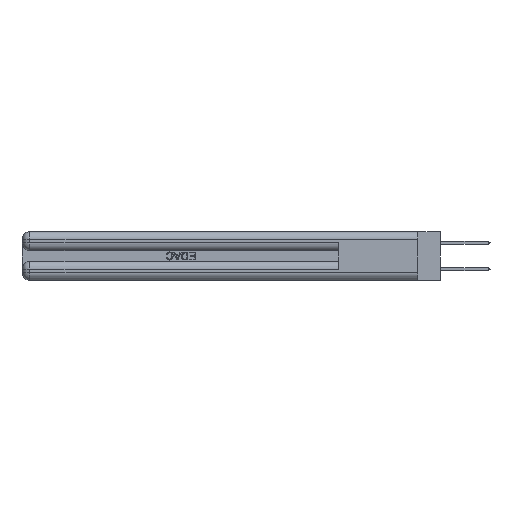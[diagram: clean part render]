
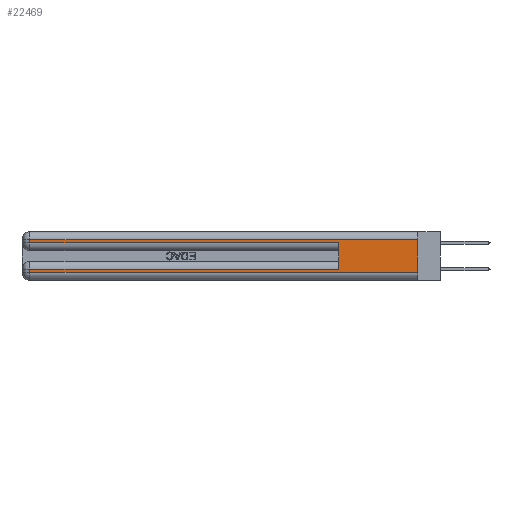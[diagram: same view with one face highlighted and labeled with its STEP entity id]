
A CAD part, left-side view. The second image highlights one B-rep face of the part: STEP entity #22469.
In plain terms, the highlighted planar face has unit normal (-1, 0, 0).
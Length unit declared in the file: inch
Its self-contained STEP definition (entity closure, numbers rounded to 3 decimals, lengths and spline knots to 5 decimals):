
#849 = DIRECTION ( 'NONE',  ( 0., 0., -1. ) ) ;
#931 = VECTOR ( 'NONE', #8853, 39.37008 ) ;
#965 = VERTEX_POINT ( 'NONE', #5379 ) ;
#1488 = CARTESIAN_POINT ( 'NONE',  ( 0., 0.6, 0.285 ) ) ;
#1806 = DIRECTION ( 'NONE',  ( 0., 1., 0. ) ) ;
#2777 = ORIENTED_EDGE ( 'NONE', *, *, #23682, .F. ) ;
#2875 = VERTEX_POINT ( 'NONE', #8921 ) ;
#2984 = DIRECTION ( 'NONE',  ( 0., 0., -1. ) ) ;
#4724 = VECTOR ( 'NONE', #29897, 39.37008 ) ;
#5170 = EDGE_CURVE ( 'NONE', #48050, #49299, #44335, .T. ) ;
#5379 = CARTESIAN_POINT ( 'NONE',  ( 0., 2.94, 0.285 ) ) ;
#5836 = CARTESIAN_POINT ( 'NONE',  ( 0., 0., 0.37 ) ) ;
#6632 = CARTESIAN_POINT ( 'NONE',  ( 0., 2.94, 0.37 ) ) ;
#6850 = VERTEX_POINT ( 'NONE', #25359 ) ;
#8327 = LINE ( 'NONE', #14644, #4724 ) ;
#8853 = DIRECTION ( 'NONE',  ( 0., 0., 1. ) ) ;
#8921 = CARTESIAN_POINT ( 'NONE',  ( 0., 2.94, 0.085 ) ) ;
#9682 = PLANE ( 'NONE',  #49146 ) ;
#9744 = LINE ( 'NONE', #6632, #49109 ) ;
#12824 = EDGE_CURVE ( 'NONE', #6850, #27339, #24992, .T. ) ;
#13044 = VECTOR ( 'NONE', #34983, 39.37008 ) ;
#13506 = DIRECTION ( 'NONE',  ( 1., 0., 0. ) ) ;
#14277 = ORIENTED_EDGE ( 'NONE', *, *, #18989, .T. ) ;
#14644 = CARTESIAN_POINT ( 'NONE',  ( 0., 0., 0.285 ) ) ;
#18989 = EDGE_CURVE ( 'NONE', #965, #36957, #8327, .T. ) ;
#19018 = ORIENTED_EDGE ( 'NONE', *, *, #34756, .F. ) ;
#19225 = EDGE_CURVE ( 'NONE', #48373, #2875, #23303, .T. ) ;
#22469 = ADVANCED_FACE ( 'NONE', ( #30700 ), #9682, .F. ) ;
#23303 = LINE ( 'NONE', #23380, #13044 ) ;
#23380 = CARTESIAN_POINT ( 'NONE',  ( 0., 0., 0.085 ) ) ;
#23419 = ORIENTED_EDGE ( 'NONE', *, *, #47193, .T. ) ;
#23682 = EDGE_CURVE ( 'NONE', #48050, #27339, #27662, .T. ) ;
#24127 = EDGE_CURVE ( 'NONE', #2875, #6850, #37663, .T. ) ;
#24497 = CARTESIAN_POINT ( 'NONE',  ( 0., 0., 0.37 ) ) ;
#24730 = CARTESIAN_POINT ( 'NONE',  ( 0., 0., 0.31 ) ) ;
#24992 = LINE ( 'NONE', #44428, #35106 ) ;
#25359 = CARTESIAN_POINT ( 'NONE',  ( 0., 2.94, 0.06 ) ) ;
#25390 = DIRECTION ( 'NONE',  ( 0., -1., 0. ) ) ;
#26011 = ORIENTED_EDGE ( 'NONE', *, *, #12824, .T. ) ;
#26036 = CARTESIAN_POINT ( 'NONE',  ( 0., 0., 0.06 ) ) ;
#26430 = VECTOR ( 'NONE', #849, 39.37008 ) ;
#27339 = VERTEX_POINT ( 'NONE', #26036 ) ;
#27483 = CARTESIAN_POINT ( 'NONE',  ( 0., 2.94, 0.37 ) ) ;
#27521 = CARTESIAN_POINT ( 'NONE',  ( 0., 0., 0.31 ) ) ;
#27662 = LINE ( 'NONE', #24497, #46615 ) ;
#28335 = DIRECTION ( 'NONE',  ( 0., 0., -1. ) ) ;
#29074 = CARTESIAN_POINT ( 'NONE',  ( 0., 0.6, 0.085 ) ) ;
#29897 = DIRECTION ( 'NONE',  ( 0., -1., 0. ) ) ;
#30271 = LINE ( 'NONE', #35562, #931 ) ;
#30700 = FACE_OUTER_BOUND ( 'NONE', #41148, .T. ) ;
#34298 = VECTOR ( 'NONE', #1806, 39.37008 ) ;
#34756 = EDGE_CURVE ( 'NONE', #48373, #36957, #30271, .T. ) ;
#34983 = DIRECTION ( 'NONE',  ( 0., 1., 0. ) ) ;
#35106 = VECTOR ( 'NONE', #25390, 39.37008 ) ;
#35562 = CARTESIAN_POINT ( 'NONE',  ( 0., 0.6, 0.145 ) ) ;
#36957 = VERTEX_POINT ( 'NONE', #1488 ) ;
#37591 = CARTESIAN_POINT ( 'NONE',  ( 0., 2.94, 0.31 ) ) ;
#37663 = LINE ( 'NONE', #27483, #26430 ) ;
#40176 = DIRECTION ( 'NONE',  ( 0., 0., -1. ) ) ;
#41148 = EDGE_LOOP ( 'NONE', ( #2777, #47633, #23419, #14277, #19018, #48604, #48106, #26011 ) ) ;
#44335 = LINE ( 'NONE', #24730, #34298 ) ;
#44428 = CARTESIAN_POINT ( 'NONE',  ( 0., 0., 0.06 ) ) ;
#46615 = VECTOR ( 'NONE', #28335, 39.37008 ) ;
#47193 = EDGE_CURVE ( 'NONE', #49299, #965, #9744, .T. ) ;
#47633 = ORIENTED_EDGE ( 'NONE', *, *, #5170, .T. ) ;
#48050 = VERTEX_POINT ( 'NONE', #27521 ) ;
#48106 = ORIENTED_EDGE ( 'NONE', *, *, #24127, .T. ) ;
#48373 = VERTEX_POINT ( 'NONE', #29074 ) ;
#48604 = ORIENTED_EDGE ( 'NONE', *, *, #19225, .T. ) ;
#49109 = VECTOR ( 'NONE', #2984, 39.37008 ) ;
#49146 = AXIS2_PLACEMENT_3D ( 'NONE', #5836, #13506, #40176 ) ;
#49299 = VERTEX_POINT ( 'NONE', #37591 ) ;
